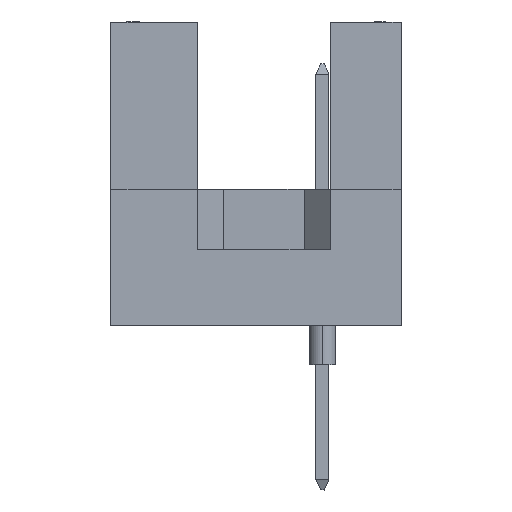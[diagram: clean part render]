
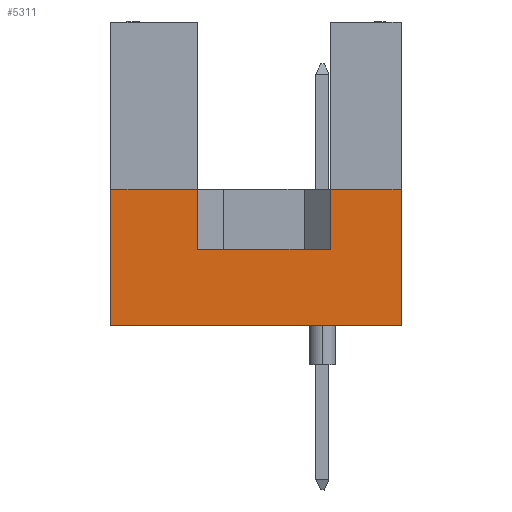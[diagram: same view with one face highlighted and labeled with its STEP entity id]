
A CAD part, left-side view. The second image highlights one B-rep face of the part: STEP entity #5311.
In plain terms, the highlighted planar face has unit normal (-1, 0, 0).
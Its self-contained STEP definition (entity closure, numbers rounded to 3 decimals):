
#352 = DIRECTION ( 'NONE',  ( 0., 0., -1. ) ) ;
#1471 = LINE ( 'NONE', #14321, #12899 ) ;
#1547 = ORIENTED_EDGE ( 'NONE', *, *, #2591, .T. ) ;
#1910 = EDGE_CURVE ( 'NONE', #3638, #4547, #14992, .T. ) ;
#2304 = CARTESIAN_POINT ( 'NONE',  ( -47.5, 11.1, 0. ) ) ;
#2465 = VERTEX_POINT ( 'NONE', #15872 ) ;
#2478 = ORIENTED_EDGE ( 'NONE', *, *, #15519, .T. ) ;
#2540 = ORIENTED_EDGE ( 'NONE', *, *, #14203, .F. ) ;
#2591 = EDGE_CURVE ( 'NONE', #6773, #13140, #9656, .T. ) ;
#2704 = CARTESIAN_POINT ( 'NONE',  ( -47.5, 11.1, 0. ) ) ;
#2735 = CARTESIAN_POINT ( 'NONE',  ( -47.5, 11.1, 0. ) ) ;
#2912 = VERTEX_POINT ( 'NONE', #4019 ) ;
#3516 = CARTESIAN_POINT ( 'NONE',  ( -47.5, 7.79, 2.9 ) ) ;
#3638 = VERTEX_POINT ( 'NONE', #2304 ) ;
#3956 = DIRECTION ( 'NONE',  ( 0., 0., 1. ) ) ;
#4019 = CARTESIAN_POINT ( 'NONE',  ( -47.5, 7.79, 2.9 ) ) ;
#4044 = CARTESIAN_POINT ( 'NONE',  ( -47.5, 2.71, 2.9 ) ) ;
#4547 = VERTEX_POINT ( 'NONE', #9858 ) ;
#4732 = VECTOR ( 'NONE', #14777, 1000. ) ;
#5016 = DIRECTION ( 'NONE',  ( 0., 0., 1. ) ) ;
#5311 = ADVANCED_FACE ( 'NONE', ( #8997 ), #9248, .F. ) ;
#5354 = EDGE_CURVE ( 'NONE', #8669, #2465, #7995, .T. ) ;
#6250 = ORIENTED_EDGE ( 'NONE', *, *, #10347, .T. ) ;
#6396 = EDGE_LOOP ( 'NONE', ( #14688, #6250, #2540, #6718, #2478, #1547, #9687, #11272 ) ) ;
#6718 = ORIENTED_EDGE ( 'NONE', *, *, #1910, .F. ) ;
#6758 = DIRECTION ( 'NONE',  ( 0., -1., 0. ) ) ;
#6773 = VERTEX_POINT ( 'NONE', #16298 ) ;
#7285 = VECTOR ( 'NONE', #3956, 1000. ) ;
#7353 = CARTESIAN_POINT ( 'NONE',  ( -47.5, 11.1, 0. ) ) ;
#7833 = DIRECTION ( 'NONE',  ( 1., 0., 0. ) ) ;
#7995 = LINE ( 'NONE', #4044, #7285 ) ;
#8078 = CARTESIAN_POINT ( 'NONE',  ( -47.5, 11.1, 5.2 ) ) ;
#8125 = VERTEX_POINT ( 'NONE', #15125 ) ;
#8169 = CARTESIAN_POINT ( 'NONE',  ( -47.5, 7.79, 2.9 ) ) ;
#8669 = VERTEX_POINT ( 'NONE', #15773 ) ;
#8997 = FACE_OUTER_BOUND ( 'NONE', #6396, .T. ) ;
#9248 = PLANE ( 'NONE',  #12375 ) ;
#9339 = DIRECTION ( 'NONE',  ( 0., -1., 0. ) ) ;
#9656 = LINE ( 'NONE', #14692, #4732 ) ;
#9687 = ORIENTED_EDGE ( 'NONE', *, *, #12687, .F. ) ;
#9858 = CARTESIAN_POINT ( 'NONE',  ( -47.5, 11.1, 5.2 ) ) ;
#10058 = VECTOR ( 'NONE', #5016, 1000. ) ;
#10061 = LINE ( 'NONE', #3516, #10058 ) ;
#10347 = EDGE_CURVE ( 'NONE', #2912, #8125, #10061, .T. ) ;
#10457 = DIRECTION ( 'NONE',  ( 0., -1., 0. ) ) ;
#10724 = VECTOR ( 'NONE', #15617, 1000. ) ;
#10862 = VECTOR ( 'NONE', #9339, 1000. ) ;
#11272 = ORIENTED_EDGE ( 'NONE', *, *, #5354, .F. ) ;
#12375 = AXIS2_PLACEMENT_3D ( 'NONE', #2704, #7833, #352 ) ;
#12687 = EDGE_CURVE ( 'NONE', #2465, #13140, #13278, .T. ) ;
#12899 = VECTOR ( 'NONE', #10457, 1000. ) ;
#13043 = LINE ( 'NONE', #8169, #10862 ) ;
#13140 = VERTEX_POINT ( 'NONE', #14355 ) ;
#13228 = LINE ( 'NONE', #2735, #15138 ) ;
#13278 = LINE ( 'NONE', #8078, #10724 ) ;
#14203 = EDGE_CURVE ( 'NONE', #4547, #8125, #1471, .T. ) ;
#14321 = CARTESIAN_POINT ( 'NONE',  ( -47.5, 11.1, 5.2 ) ) ;
#14355 = CARTESIAN_POINT ( 'NONE',  ( -47.5, 0., 5.2 ) ) ;
#14603 = VECTOR ( 'NONE', #15075, 1000. ) ;
#14688 = ORIENTED_EDGE ( 'NONE', *, *, #15953, .F. ) ;
#14692 = CARTESIAN_POINT ( 'NONE',  ( -47.5, 0., 0. ) ) ;
#14777 = DIRECTION ( 'NONE',  ( 0., 0., 1. ) ) ;
#14992 = LINE ( 'NONE', #7353, #14603 ) ;
#15075 = DIRECTION ( 'NONE',  ( 0., 0., 1. ) ) ;
#15125 = CARTESIAN_POINT ( 'NONE',  ( -47.5, 7.79, 5.2 ) ) ;
#15138 = VECTOR ( 'NONE', #6758, 1000. ) ;
#15519 = EDGE_CURVE ( 'NONE', #3638, #6773, #13228, .T. ) ;
#15617 = DIRECTION ( 'NONE',  ( 0., -1., 0. ) ) ;
#15773 = CARTESIAN_POINT ( 'NONE',  ( -47.5, 2.71, 2.9 ) ) ;
#15872 = CARTESIAN_POINT ( 'NONE',  ( -47.5, 2.71, 5.2 ) ) ;
#15953 = EDGE_CURVE ( 'NONE', #2912, #8669, #13043, .T. ) ;
#16298 = CARTESIAN_POINT ( 'NONE',  ( -47.5, 0., 0. ) ) ;
